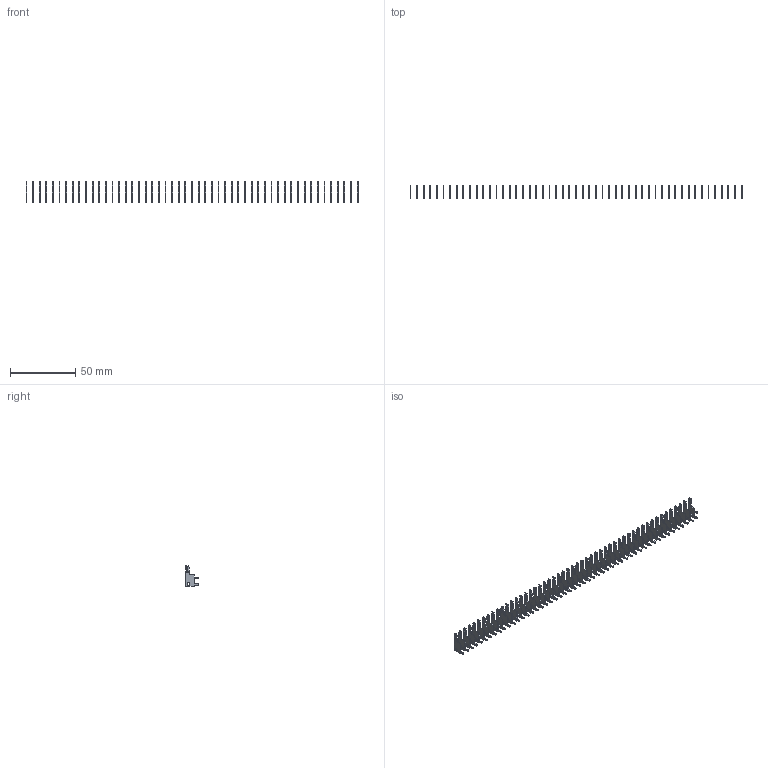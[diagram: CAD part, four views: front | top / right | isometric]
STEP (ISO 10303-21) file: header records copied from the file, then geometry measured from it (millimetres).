
FILE_DESCRIPTION (( 'STEP AP203' ), '1' );
FILE_NAME ('105-051-201-200.STEP', '2020-04-08T00:28:03', ( '' ), ( '' ), 'SwSTEP 2.0', 'SolidWorks 2016', '' );
FILE_SCHEMA (( 'CONFIG_CONTROL_DESIGN' ));
Length unit declared in the file: inch
Products named in the file (2): 100-290-001_100-290-201; 105-051-201-200
Assembly tree (51 placements, depth 2):
  105-051-201-200
    100-290-001_100-290-201  x51
Bounding box: 254.63 x 9.7 x 15.88 mm (x, y, z)
Volume: 2511.3 mm3; surface area: 10248 mm2
Topology: 51 solids, 51 shells, 1785 faces, 5049 edges, 3366 vertices
Faces by surface type: plane 1275, cylinder 510
Entity records: 2937 total; most frequent: DIRECTION 293, CARTESIAN_POINT 266, ORIENTED_EDGE 198, DATE_AND_TIME 112, LOCAL_TIME 112, CALENDAR_DATE 112, COORDINATED_UNIVERSAL_TIME_OFFSET 112, AXIS2_PLACEMENT_3D 109
